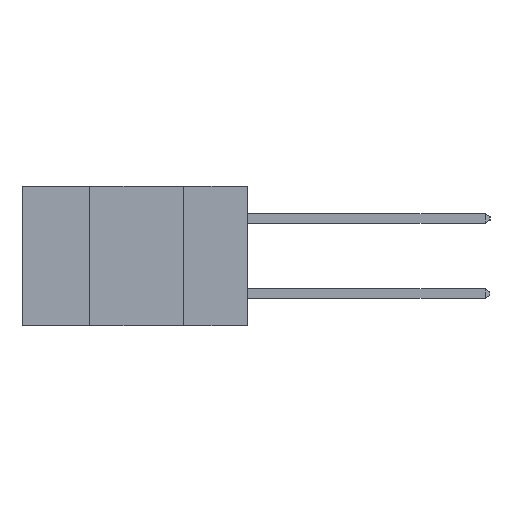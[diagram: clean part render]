
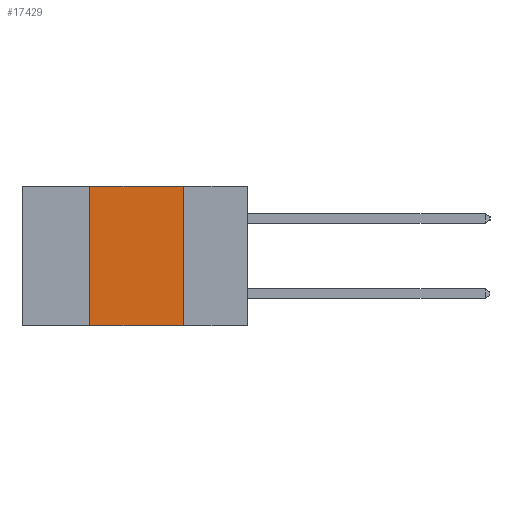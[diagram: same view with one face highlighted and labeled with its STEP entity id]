
A CAD part, left-side view. The second image highlights one B-rep face of the part: STEP entity #17429.
In plain terms, the highlighted planar face has unit normal (-1, 0, 0).
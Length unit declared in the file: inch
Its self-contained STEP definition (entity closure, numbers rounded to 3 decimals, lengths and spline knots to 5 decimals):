
#765 = CARTESIAN_POINT ( 'NONE',  ( 0., 0.6, 0. ) ) ;
#1296 = VECTOR ( 'NONE', #7309, 39.37008 ) ;
#1744 = CARTESIAN_POINT ( 'NONE',  ( 0., 0.17, 0. ) ) ;
#2230 = ORIENTED_EDGE ( 'NONE', *, *, #14723, .F. ) ;
#2280 = DIRECTION ( 'NONE',  ( 0., 0., -1. ) ) ;
#2742 = LINE ( 'NONE', #10724, #10356 ) ;
#2865 = EDGE_CURVE ( 'NONE', #9641, #4751, #2742, .T. ) ;
#3063 = AXIS2_PLACEMENT_3D ( 'NONE', #765, #11332, #2280 ) ;
#3855 = EDGE_CURVE ( 'NONE', #9641, #17737, #15531, .T. ) ;
#4101 = VECTOR ( 'NONE', #11742, 39.37008 ) ;
#4751 = VERTEX_POINT ( 'NONE', #18773 ) ;
#4789 = VECTOR ( 'NONE', #18628, 39.37008 ) ;
#5921 = EDGE_LOOP ( 'NONE', ( #9581, #2230, #18576, #15406 ) ) ;
#7309 = DIRECTION ( 'NONE',  ( 0., -1., 0. ) ) ;
#8907 = LINE ( 'NONE', #14230, #4789 ) ;
#8983 = EDGE_CURVE ( 'NONE', #10109, #4751, #8907, .T. ) ;
#9581 = ORIENTED_EDGE ( 'NONE', *, *, #8983, .F. ) ;
#9641 = VERTEX_POINT ( 'NONE', #9834 ) ;
#9834 = CARTESIAN_POINT ( 'NONE',  ( 0., 0.42, -0.37 ) ) ;
#10109 = VERTEX_POINT ( 'NONE', #1744 ) ;
#10356 = VECTOR ( 'NONE', #10771, 39.37008 ) ;
#10724 = CARTESIAN_POINT ( 'NONE',  ( 0., 0.6, -0.37 ) ) ;
#10771 = DIRECTION ( 'NONE',  ( 0., -1., 0. ) ) ;
#11132 = CARTESIAN_POINT ( 'NONE',  ( 0., 0.42, 0. ) ) ;
#11332 = DIRECTION ( 'NONE',  ( 1., 0., 0. ) ) ;
#11742 = DIRECTION ( 'NONE',  ( 0., 0., 1. ) ) ;
#11933 = CARTESIAN_POINT ( 'NONE',  ( 0., 0.42, 0. ) ) ;
#14230 = CARTESIAN_POINT ( 'NONE',  ( 0., 0.17, 0. ) ) ;
#14410 = FACE_OUTER_BOUND ( 'NONE', #5921, .T. ) ;
#14665 = CARTESIAN_POINT ( 'NONE',  ( 0., 0.6, 0. ) ) ;
#14723 = EDGE_CURVE ( 'NONE', #17737, #10109, #18024, .T. ) ;
#15406 = ORIENTED_EDGE ( 'NONE', *, *, #2865, .T. ) ;
#15531 = LINE ( 'NONE', #11132, #4101 ) ;
#17098 = PLANE ( 'NONE',  #3063 ) ;
#17429 = ADVANCED_FACE ( 'NONE', ( #14410 ), #17098, .F. ) ;
#17737 = VERTEX_POINT ( 'NONE', #11933 ) ;
#18024 = LINE ( 'NONE', #14665, #1296 ) ;
#18576 = ORIENTED_EDGE ( 'NONE', *, *, #3855, .F. ) ;
#18628 = DIRECTION ( 'NONE',  ( 0., 0., -1. ) ) ;
#18773 = CARTESIAN_POINT ( 'NONE',  ( 0., 0.17, -0.37 ) ) ;
